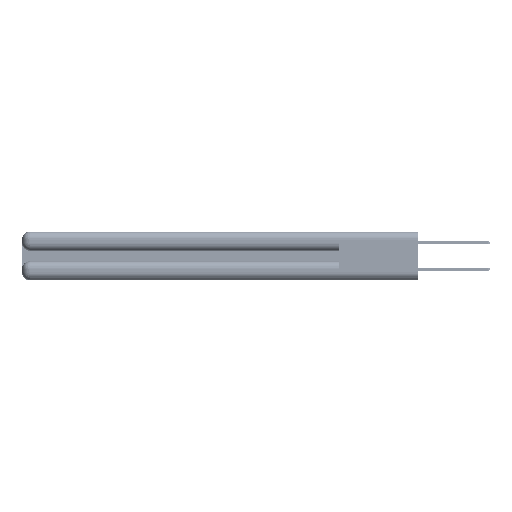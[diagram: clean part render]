
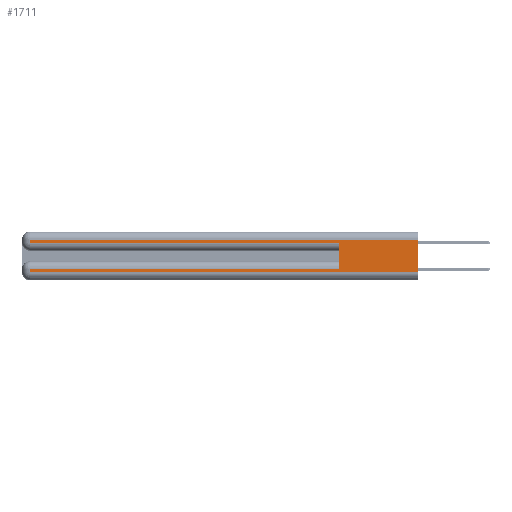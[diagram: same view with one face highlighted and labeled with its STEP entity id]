
A CAD part, left-side view. The second image highlights one B-rep face of the part: STEP entity #1711.
In plain terms, the highlighted planar face has unit normal (-1, 0, 0).
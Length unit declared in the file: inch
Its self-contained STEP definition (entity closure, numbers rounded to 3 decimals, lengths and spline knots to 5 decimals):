
#255 = VECTOR ( 'NONE', #14947, 39.37008 ) ;
#922 = CARTESIAN_POINT ( 'NONE',  ( 0., 2.94, 0.085 ) ) ;
#1711 = ADVANCED_FACE ( 'NONE', ( #9898 ), #3924, .F. ) ;
#3447 = LINE ( 'NONE', #23539, #21684 ) ;
#3924 = PLANE ( 'NONE',  #9027 ) ;
#3951 = VERTEX_POINT ( 'NONE', #22221 ) ;
#4068 = VERTEX_POINT ( 'NONE', #922 ) ;
#4327 = EDGE_CURVE ( 'NONE', #4068, #6536, #4359, .T. ) ;
#4359 = LINE ( 'NONE', #42104, #42751 ) ;
#5403 = VECTOR ( 'NONE', #13155, 39.37008 ) ;
#5912 = CARTESIAN_POINT ( 'NONE',  ( 0., 0., 0.285 ) ) ;
#6536 = VERTEX_POINT ( 'NONE', #27235 ) ;
#6850 = ORIENTED_EDGE ( 'NONE', *, *, #25406, .T. ) ;
#7238 = EDGE_CURVE ( 'NONE', #14058, #28602, #3447, .T. ) ;
#8386 = EDGE_CURVE ( 'NONE', #28602, #41144, #39322, .T. ) ;
#8676 = LINE ( 'NONE', #45996, #41658 ) ;
#9027 = AXIS2_PLACEMENT_3D ( 'NONE', #55659, #29764, #21825 ) ;
#9354 = DIRECTION ( 'NONE',  ( 0., 1., 0. ) ) ;
#9898 = FACE_OUTER_BOUND ( 'NONE', #22275, .T. ) ;
#10836 = LINE ( 'NONE', #15713, #41126 ) ;
#12836 = CARTESIAN_POINT ( 'NONE',  ( 0., 0.6, 0.285 ) ) ;
#13155 = DIRECTION ( 'NONE',  ( 0., -1., 0. ) ) ;
#13551 = CARTESIAN_POINT ( 'NONE',  ( 0., 0., 0.06 ) ) ;
#14058 = VERTEX_POINT ( 'NONE', #31267 ) ;
#14947 = DIRECTION ( 'NONE',  ( 0., -1., 0. ) ) ;
#15713 = CARTESIAN_POINT ( 'NONE',  ( 0., 0., 0.37 ) ) ;
#16139 = DIRECTION ( 'NONE',  ( 0., 0., -1. ) ) ;
#17465 = CARTESIAN_POINT ( 'NONE',  ( 0., 0., 0.06 ) ) ;
#18934 = ORIENTED_EDGE ( 'NONE', *, *, #39546, .T. ) ;
#19862 = VERTEX_POINT ( 'NONE', #13551 ) ;
#20435 = VERTEX_POINT ( 'NONE', #39080 ) ;
#21684 = VECTOR ( 'NONE', #45148, 39.37008 ) ;
#21825 = DIRECTION ( 'NONE',  ( 0., 0., -1. ) ) ;
#22221 = CARTESIAN_POINT ( 'NONE',  ( 0., 0.6, 0.085 ) ) ;
#22275 = EDGE_LOOP ( 'NONE', ( #38974, #18934, #23565, #29728, #42986, #6850, #26869, #54366 ) ) ;
#23539 = CARTESIAN_POINT ( 'NONE',  ( 0., 2.94, 0.37 ) ) ;
#23565 = ORIENTED_EDGE ( 'NONE', *, *, #7238, .T. ) ;
#25406 = EDGE_CURVE ( 'NONE', #3951, #4068, #31884, .T. ) ;
#26869 = ORIENTED_EDGE ( 'NONE', *, *, #4327, .T. ) ;
#26983 = LINE ( 'NONE', #17465, #5403 ) ;
#27235 = CARTESIAN_POINT ( 'NONE',  ( 0., 2.94, 0.06 ) ) ;
#27727 = CARTESIAN_POINT ( 'NONE',  ( 0., 0.6, 0.145 ) ) ;
#28602 = VERTEX_POINT ( 'NONE', #31206 ) ;
#29728 = ORIENTED_EDGE ( 'NONE', *, *, #8386, .T. ) ;
#29764 = DIRECTION ( 'NONE',  ( 1., 0., 0. ) ) ;
#31206 = CARTESIAN_POINT ( 'NONE',  ( 0., 2.94, 0.285 ) ) ;
#31267 = CARTESIAN_POINT ( 'NONE',  ( 0., 2.94, 0.31 ) ) ;
#31884 = LINE ( 'NONE', #52240, #41303 ) ;
#33826 = EDGE_CURVE ( 'NONE', #3951, #41144, #48465, .T. ) ;
#34482 = EDGE_CURVE ( 'NONE', #20435, #19862, #10836, .T. ) ;
#38974 = ORIENTED_EDGE ( 'NONE', *, *, #34482, .F. ) ;
#39080 = CARTESIAN_POINT ( 'NONE',  ( 0., 0., 0.31 ) ) ;
#39322 = LINE ( 'NONE', #5912, #255 ) ;
#39546 = EDGE_CURVE ( 'NONE', #20435, #14058, #8676, .T. ) ;
#40498 = DIRECTION ( 'NONE',  ( 0., 0., 1. ) ) ;
#41126 = VECTOR ( 'NONE', #47694, 39.37008 ) ;
#41144 = VERTEX_POINT ( 'NONE', #12836 ) ;
#41303 = VECTOR ( 'NONE', #9354, 39.37008 ) ;
#41658 = VECTOR ( 'NONE', #50149, 39.37008 ) ;
#42104 = CARTESIAN_POINT ( 'NONE',  ( 0., 2.94, 0.37 ) ) ;
#42751 = VECTOR ( 'NONE', #16139, 39.37008 ) ;
#42986 = ORIENTED_EDGE ( 'NONE', *, *, #33826, .F. ) ;
#45148 = DIRECTION ( 'NONE',  ( 0., 0., -1. ) ) ;
#45996 = CARTESIAN_POINT ( 'NONE',  ( 0., 0., 0.31 ) ) ;
#47694 = DIRECTION ( 'NONE',  ( 0., 0., -1. ) ) ;
#48465 = LINE ( 'NONE', #27727, #52533 ) ;
#50149 = DIRECTION ( 'NONE',  ( 0., 1., 0. ) ) ;
#51884 = EDGE_CURVE ( 'NONE', #6536, #19862, #26983, .T. ) ;
#52240 = CARTESIAN_POINT ( 'NONE',  ( 0., 0., 0.085 ) ) ;
#52533 = VECTOR ( 'NONE', #40498, 39.37008 ) ;
#54366 = ORIENTED_EDGE ( 'NONE', *, *, #51884, .T. ) ;
#55659 = CARTESIAN_POINT ( 'NONE',  ( 0., 0., 0.37 ) ) ;
